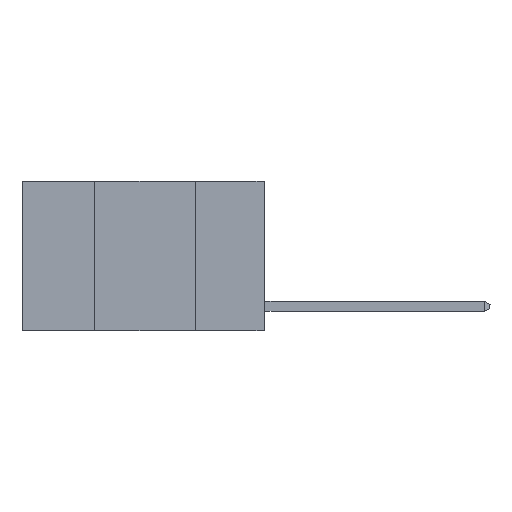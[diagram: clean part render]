
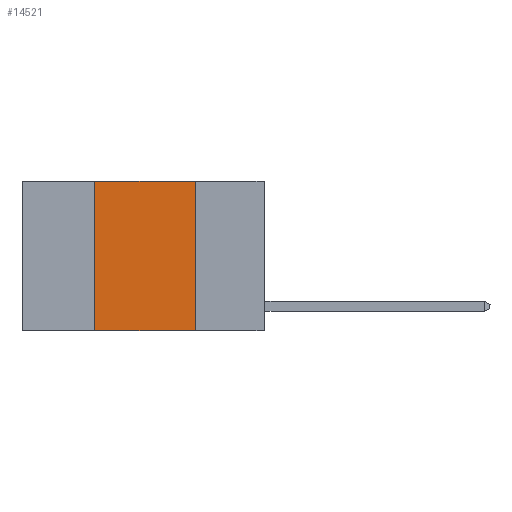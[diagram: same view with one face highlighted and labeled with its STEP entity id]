
A CAD part, left-side view. The second image highlights one B-rep face of the part: STEP entity #14521.
In plain terms, the highlighted planar face has unit normal (-1, 0, 0).
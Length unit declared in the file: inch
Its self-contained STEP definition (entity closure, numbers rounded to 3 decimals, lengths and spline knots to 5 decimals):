
#507 = PLANE ( 'NONE',  #8484 ) ;
#674 = DIRECTION ( 'NONE',  ( 0., -1., 0. ) ) ;
#1176 = CARTESIAN_POINT ( 'NONE',  ( 0., 0.42, 0. ) ) ;
#1262 = CARTESIAN_POINT ( 'NONE',  ( 0., 0.42, 0. ) ) ;
#1864 = DIRECTION ( 'NONE',  ( 1., 0., 0. ) ) ;
#2904 = ORIENTED_EDGE ( 'NONE', *, *, #6849, .T. ) ;
#3078 = VERTEX_POINT ( 'NONE', #16524 ) ;
#4423 = LINE ( 'NONE', #8915, #10476 ) ;
#6043 = DIRECTION ( 'NONE',  ( 0., -1., 0. ) ) ;
#6290 = CARTESIAN_POINT ( 'NONE',  ( 0., 0.17, 0. ) ) ;
#6456 = EDGE_CURVE ( 'NONE', #12593, #11627, #4423, .T. ) ;
#6843 = VECTOR ( 'NONE', #10758, 39.37008 ) ;
#6849 = EDGE_CURVE ( 'NONE', #3078, #17276, #15909, .T. ) ;
#8331 = VECTOR ( 'NONE', #16198, 39.37008 ) ;
#8471 = CARTESIAN_POINT ( 'NONE',  ( 0., 0.17, -0.37 ) ) ;
#8484 = AXIS2_PLACEMENT_3D ( 'NONE', #10103, #1864, #10170 ) ;
#8915 = CARTESIAN_POINT ( 'NONE',  ( 0., 0.6, 0. ) ) ;
#9940 = ORIENTED_EDGE ( 'NONE', *, *, #12436, .F. ) ;
#10103 = CARTESIAN_POINT ( 'NONE',  ( 0., 0.6, 0. ) ) ;
#10170 = DIRECTION ( 'NONE',  ( 0., 0., -1. ) ) ;
#10430 = CARTESIAN_POINT ( 'NONE',  ( 0., 0.17, 0. ) ) ;
#10476 = VECTOR ( 'NONE', #674, 39.37008 ) ;
#10758 = DIRECTION ( 'NONE',  ( 0., 0., 1. ) ) ;
#11627 = VERTEX_POINT ( 'NONE', #6290 ) ;
#11659 = EDGE_CURVE ( 'NONE', #3078, #12593, #13375, .T. ) ;
#12436 = EDGE_CURVE ( 'NONE', #11627, #17276, #12668, .T. ) ;
#12593 = VERTEX_POINT ( 'NONE', #1262 ) ;
#12668 = LINE ( 'NONE', #10430, #8331 ) ;
#12857 = VECTOR ( 'NONE', #6043, 39.37008 ) ;
#13375 = LINE ( 'NONE', #1176, #6843 ) ;
#14521 = ADVANCED_FACE ( 'NONE', ( #16307 ), #507, .F. ) ;
#14827 = ORIENTED_EDGE ( 'NONE', *, *, #6456, .F. ) ;
#15830 = CARTESIAN_POINT ( 'NONE',  ( 0., 0.6, -0.37 ) ) ;
#15909 = LINE ( 'NONE', #15830, #12857 ) ;
#16027 = EDGE_LOOP ( 'NONE', ( #9940, #14827, #16335, #2904 ) ) ;
#16198 = DIRECTION ( 'NONE',  ( 0., 0., -1. ) ) ;
#16307 = FACE_OUTER_BOUND ( 'NONE', #16027, .T. ) ;
#16335 = ORIENTED_EDGE ( 'NONE', *, *, #11659, .F. ) ;
#16524 = CARTESIAN_POINT ( 'NONE',  ( 0., 0.42, -0.37 ) ) ;
#17276 = VERTEX_POINT ( 'NONE', #8471 ) ;
